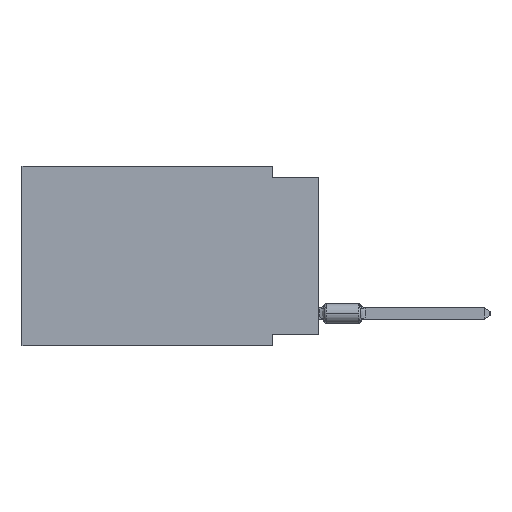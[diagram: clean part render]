
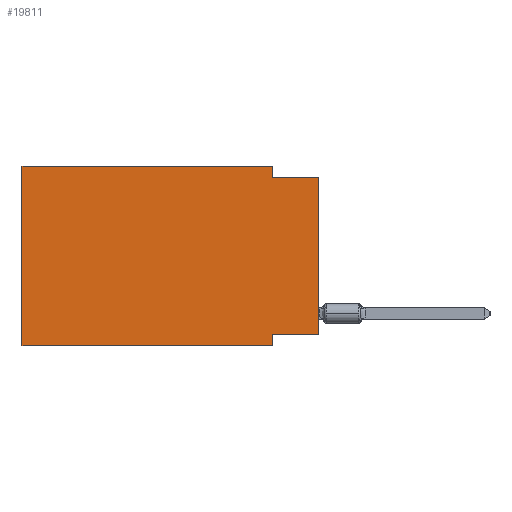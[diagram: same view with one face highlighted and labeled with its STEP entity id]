
A CAD part, left-side view. The second image highlights one B-rep face of the part: STEP entity #19811.
In plain terms, the highlighted planar face has unit normal (-1, 0, 0).
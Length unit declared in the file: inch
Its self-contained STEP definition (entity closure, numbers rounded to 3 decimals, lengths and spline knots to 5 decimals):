
#1169 = CARTESIAN_POINT ( 'NONE',  ( 0., 0.645, 0. ) ) ;
#1479 = VERTEX_POINT ( 'NONE', #3256 ) ;
#1765 = VECTOR ( 'NONE', #40272, 39.37008 ) ;
#1864 = CARTESIAN_POINT ( 'NONE',  ( 0., 0.645, -0.39 ) ) ;
#3256 = CARTESIAN_POINT ( 'NONE',  ( 0., 0., -0.365 ) ) ;
#4372 = DIRECTION ( 'NONE',  ( 1., 0., 0. ) ) ;
#7167 = VECTOR ( 'NONE', #38132, 39.37008 ) ;
#7909 = CARTESIAN_POINT ( 'NONE',  ( 0., 0.1, -0.365 ) ) ;
#10161 = VERTEX_POINT ( 'NONE', #16392 ) ;
#11804 = LINE ( 'NONE', #30911, #38556 ) ;
#12016 = ORIENTED_EDGE ( 'NONE', *, *, #39632, .T. ) ;
#13353 = VECTOR ( 'NONE', #32680, 39.37008 ) ;
#13970 = EDGE_CURVE ( 'NONE', #40796, #50109, #28030, .T. ) ;
#14362 = CARTESIAN_POINT ( 'NONE',  ( 0., 0., -0.365 ) ) ;
#15030 = ORIENTED_EDGE ( 'NONE', *, *, #57660, .T. ) ;
#15087 = VECTOR ( 'NONE', #25974, 39.37008 ) ;
#15228 = VECTOR ( 'NONE', #39745, 39.37008 ) ;
#15429 = ORIENTED_EDGE ( 'NONE', *, *, #13970, .F. ) ;
#15507 = DIRECTION ( 'NONE',  ( 0., 0., -1. ) ) ;
#16392 = CARTESIAN_POINT ( 'NONE',  ( 0., 0.1, -0.39 ) ) ;
#16614 = LINE ( 'NONE', #1864, #13353 ) ;
#17091 = ORIENTED_EDGE ( 'NONE', *, *, #35232, .F. ) ;
#17378 = LINE ( 'NONE', #37808, #7167 ) ;
#17782 = EDGE_CURVE ( 'NONE', #1479, #46642, #59553, .T. ) ;
#18093 = VERTEX_POINT ( 'NONE', #22914 ) ;
#19811 = ADVANCED_FACE ( 'NONE', ( #35188 ), #39877, .F. ) ;
#19851 = CARTESIAN_POINT ( 'NONE',  ( 0., 0., 0. ) ) ;
#22914 = CARTESIAN_POINT ( 'NONE',  ( 0., 0.645, -0.39 ) ) ;
#24478 = CARTESIAN_POINT ( 'NONE',  ( 0., 0.645, 0. ) ) ;
#24681 = LINE ( 'NONE', #54477, #15228 ) ;
#25974 = DIRECTION ( 'NONE',  ( 0., 0., 1. ) ) ;
#27067 = AXIS2_PLACEMENT_3D ( 'NONE', #24478, #4372, #64975 ) ;
#27395 = ORIENTED_EDGE ( 'NONE', *, *, #58752, .F. ) ;
#28030 = LINE ( 'NONE', #48115, #40245 ) ;
#29104 = DIRECTION ( 'NONE',  ( 0., 1., 0. ) ) ;
#30911 = CARTESIAN_POINT ( 'NONE',  ( 0., 0.1, 0. ) ) ;
#31168 = VERTEX_POINT ( 'NONE', #43068 ) ;
#31179 = VERTEX_POINT ( 'NONE', #34036 ) ;
#31449 = EDGE_LOOP ( 'NONE', ( #15030, #15429, #59340, #27395, #63730, #12016, #17091, #36219 ) ) ;
#32680 = DIRECTION ( 'NONE',  ( 0., -1., 0. ) ) ;
#33128 = EDGE_CURVE ( 'NONE', #31179, #40796, #11804, .T. ) ;
#34036 = CARTESIAN_POINT ( 'NONE',  ( 0., 0.1, 0. ) ) ;
#35188 = FACE_OUTER_BOUND ( 'NONE', #31449, .T. ) ;
#35232 = EDGE_CURVE ( 'NONE', #46642, #10161, #24681, .T. ) ;
#36219 = ORIENTED_EDGE ( 'NONE', *, *, #17782, .F. ) ;
#37133 = CARTESIAN_POINT ( 'NONE',  ( 0., 0.1, -0.025 ) ) ;
#37808 = CARTESIAN_POINT ( 'NONE',  ( 0., 0.645, 0. ) ) ;
#38132 = DIRECTION ( 'NONE',  ( 0., -1., 0. ) ) ;
#38556 = VECTOR ( 'NONE', #15507, 39.37008 ) ;
#39632 = EDGE_CURVE ( 'NONE', #18093, #10161, #16614, .T. ) ;
#39745 = DIRECTION ( 'NONE',  ( 0., 0., -1. ) ) ;
#39877 = PLANE ( 'NONE',  #27067 ) ;
#40245 = VECTOR ( 'NONE', #43745, 39.37008 ) ;
#40272 = DIRECTION ( 'NONE',  ( 0., 0., 1. ) ) ;
#40796 = VERTEX_POINT ( 'NONE', #37133 ) ;
#43068 = CARTESIAN_POINT ( 'NONE',  ( 0., 0.645, 0. ) ) ;
#43745 = DIRECTION ( 'NONE',  ( 0., -1., 0. ) ) ;
#46642 = VERTEX_POINT ( 'NONE', #7909 ) ;
#48115 = CARTESIAN_POINT ( 'NONE',  ( 0., 0., -0.025 ) ) ;
#48161 = EDGE_CURVE ( 'NONE', #18093, #31168, #62776, .T. ) ;
#50109 = VERTEX_POINT ( 'NONE', #60328 ) ;
#54477 = CARTESIAN_POINT ( 'NONE',  ( 0., 0.1, -0.39 ) ) ;
#57539 = VECTOR ( 'NONE', #29104, 39.37008 ) ;
#57660 = EDGE_CURVE ( 'NONE', #1479, #50109, #65697, .T. ) ;
#58752 = EDGE_CURVE ( 'NONE', #31168, #31179, #17378, .T. ) ;
#59340 = ORIENTED_EDGE ( 'NONE', *, *, #33128, .F. ) ;
#59553 = LINE ( 'NONE', #14362, #57539 ) ;
#60328 = CARTESIAN_POINT ( 'NONE',  ( 0., 0., -0.025 ) ) ;
#62776 = LINE ( 'NONE', #1169, #15087 ) ;
#63730 = ORIENTED_EDGE ( 'NONE', *, *, #48161, .F. ) ;
#64975 = DIRECTION ( 'NONE',  ( 0., 0., -1. ) ) ;
#65697 = LINE ( 'NONE', #19851, #1765 ) ;
